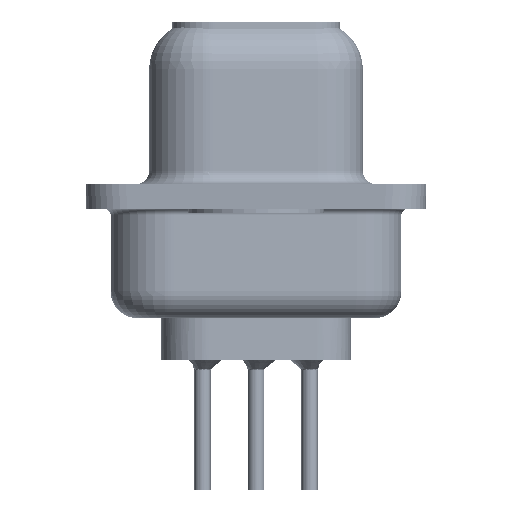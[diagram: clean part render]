
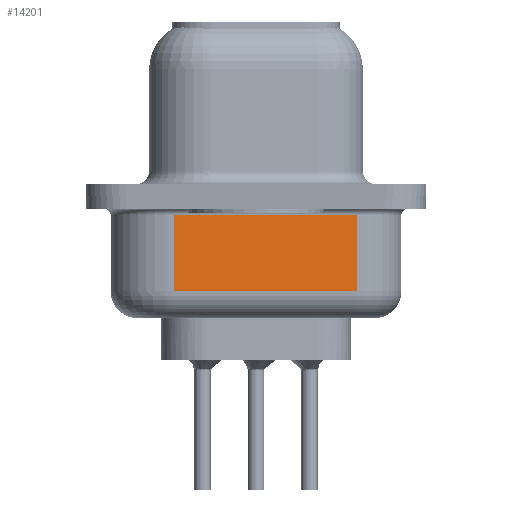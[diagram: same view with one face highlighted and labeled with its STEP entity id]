
A CAD part, left-side view. The second image highlights one B-rep face of the part: STEP entity #14201.
In plain terms, the highlighted planar face has unit normal (-0.985, -0.174, 0).
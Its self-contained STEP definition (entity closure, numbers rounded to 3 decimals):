
#244 = CARTESIAN_POINT ( 'NONE',  ( 3., 3.028, -3.5 ) ) ;
#377 = EDGE_LOOP ( 'NONE', ( #36032, #25291, #7892, #31200 ) ) ;
#1945 = LINE ( 'NONE', #25142, #20442 ) ;
#2829 = DIRECTION ( 'NONE',  ( -0.174, 0.985, 0. ) ) ;
#4253 = EDGE_CURVE ( 'NONE', #37616, #34043, #34930, .T. ) ;
#5567 = DIRECTION ( 'NONE',  ( 0., 0., 1. ) ) ;
#5658 = DIRECTION ( 'NONE',  ( 0.174, -0.985, 0. ) ) ;
#6574 = VECTOR ( 'NONE', #5567, 1000. ) ;
#6980 = DIRECTION ( 'NONE',  ( 0., 0., 1. ) ) ;
#7892 = ORIENTED_EDGE ( 'NONE', *, *, #14919, .T. ) ;
#12542 = VERTEX_POINT ( 'NONE', #32185 ) ;
#13097 = CARTESIAN_POINT ( 'NONE',  ( 3., 3.028, -0.7 ) ) ;
#13521 = AXIS2_PLACEMENT_3D ( 'NONE', #29875, #38168, #2829 ) ;
#13923 = CARTESIAN_POINT ( 'NONE',  ( 3., 3.028, -4.5 ) ) ;
#14201 = ADVANCED_FACE ( 'NONE', ( #26964 ), #29300, .F. ) ;
#14919 = EDGE_CURVE ( 'NONE', #29024, #12542, #1945, .T. ) ;
#17998 = LINE ( 'NONE', #13097, #20270 ) ;
#20270 = VECTOR ( 'NONE', #29740, 1000. ) ;
#20442 = VECTOR ( 'NONE', #6980, 1000. ) ;
#20790 = CARTESIAN_POINT ( 'NONE',  ( 4.191, -3.722, -3.5 ) ) ;
#25142 = CARTESIAN_POINT ( 'NONE',  ( 4.191, -3.722, -4.5 ) ) ;
#25291 = ORIENTED_EDGE ( 'NONE', *, *, #31714, .T. ) ;
#26964 = FACE_OUTER_BOUND ( 'NONE', #377, .T. ) ;
#29024 = VERTEX_POINT ( 'NONE', #20790 ) ;
#29300 = PLANE ( 'NONE',  #13521 ) ;
#29740 = DIRECTION ( 'NONE',  ( -0.174, 0.985, 0. ) ) ;
#29875 = CARTESIAN_POINT ( 'NONE',  ( 3., 3.028, -4.5 ) ) ;
#30047 = CARTESIAN_POINT ( 'NONE',  ( 3., 3.028, -3.5 ) ) ;
#31200 = ORIENTED_EDGE ( 'NONE', *, *, #37168, .T. ) ;
#31700 = VECTOR ( 'NONE', #5658, 1000. ) ;
#31714 = EDGE_CURVE ( 'NONE', #37616, #29024, #32135, .T. ) ;
#32135 = LINE ( 'NONE', #244, #31700 ) ;
#32185 = CARTESIAN_POINT ( 'NONE',  ( 4.191, -3.722, -0.7 ) ) ;
#34043 = VERTEX_POINT ( 'NONE', #35576 ) ;
#34930 = LINE ( 'NONE', #13923, #6574 ) ;
#35576 = CARTESIAN_POINT ( 'NONE',  ( 3., 3.028, -0.7 ) ) ;
#36032 = ORIENTED_EDGE ( 'NONE', *, *, #4253, .F. ) ;
#37168 = EDGE_CURVE ( 'NONE', #12542, #34043, #17998, .T. ) ;
#37616 = VERTEX_POINT ( 'NONE', #30047 ) ;
#38168 = DIRECTION ( 'NONE',  ( 0.985, 0.174, 0. ) ) ;
